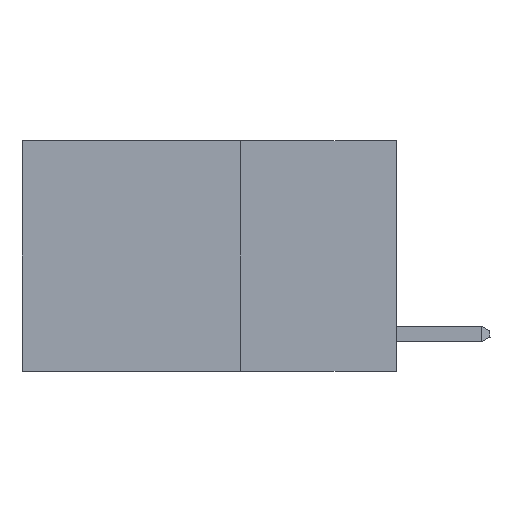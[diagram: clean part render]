
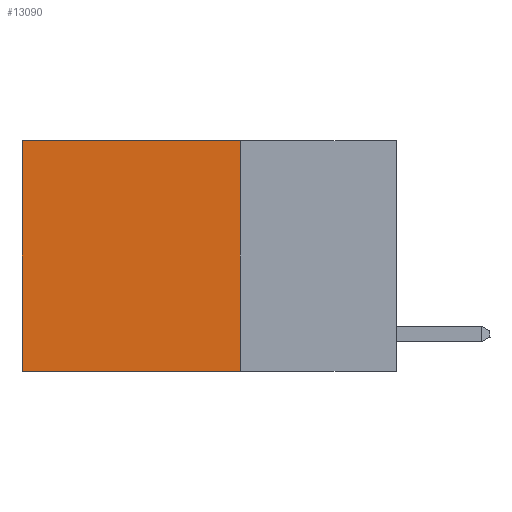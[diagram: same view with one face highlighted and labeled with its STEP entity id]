
A CAD part, left-side view. The second image highlights one B-rep face of the part: STEP entity #13090.
In plain terms, the highlighted planar face has unit normal (-1, 0, 0).
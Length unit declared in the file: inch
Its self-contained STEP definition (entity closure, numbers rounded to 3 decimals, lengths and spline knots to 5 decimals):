
#1786 = EDGE_CURVE ( 'NONE', #17122, #5156, #8942, .T. ) ;
#2832 = ORIENTED_EDGE ( 'NONE', *, *, #1786, .F. ) ;
#2873 = VECTOR ( 'NONE', #19897, 39.37008 ) ;
#3058 = LINE ( 'NONE', #7512, #3619 ) ;
#3619 = VECTOR ( 'NONE', #20273, 39.37008 ) ;
#3676 = CARTESIAN_POINT ( 'NONE',  ( 0.2625, 0.25, 0. ) ) ;
#3737 = VERTEX_POINT ( 'NONE', #13297 ) ;
#4144 = CARTESIAN_POINT ( 'NONE',  ( 0.2625, 0.25, 0. ) ) ;
#4507 = VECTOR ( 'NONE', #12484, 39.37008 ) ;
#5156 = VERTEX_POINT ( 'NONE', #11385 ) ;
#7353 = LINE ( 'NONE', #3676, #2873 ) ;
#7491 = DIRECTION ( 'NONE',  ( 0., 0., -1. ) ) ;
#7512 = CARTESIAN_POINT ( 'NONE',  ( 0.2625, 0.6, 0. ) ) ;
#7593 = VECTOR ( 'NONE', #7491, 39.37008 ) ;
#8550 = DIRECTION ( 'NONE',  ( 1., 0., 0. ) ) ;
#8942 = LINE ( 'NONE', #10857, #4507 ) ;
#10551 = CARTESIAN_POINT ( 'NONE',  ( 0.2625, 0.25, 0. ) ) ;
#10857 = CARTESIAN_POINT ( 'NONE',  ( 0.2625, 0.25, -0.37 ) ) ;
#11159 = ORIENTED_EDGE ( 'NONE', *, *, #13392, .T. ) ;
#11385 = CARTESIAN_POINT ( 'NONE',  ( 0.2625, 0.6, -0.37 ) ) ;
#11664 = ORIENTED_EDGE ( 'NONE', *, *, #11959, .F. ) ;
#11944 = LINE ( 'NONE', #4144, #7593 ) ;
#11959 = EDGE_CURVE ( 'NONE', #16475, #17122, #11944, .T. ) ;
#12484 = DIRECTION ( 'NONE',  ( 0., 1., 0. ) ) ;
#13090 = ADVANCED_FACE ( 'NONE', ( #13167 ), #18098, .F. ) ;
#13167 = FACE_OUTER_BOUND ( 'NONE', #14002, .T. ) ;
#13297 = CARTESIAN_POINT ( 'NONE',  ( 0.2625, 0.6, 0. ) ) ;
#13392 = EDGE_CURVE ( 'NONE', #3737, #5156, #3058, .T. ) ;
#14002 = EDGE_LOOP ( 'NONE', ( #11159, #2832, #11664, #20062 ) ) ;
#16475 = VERTEX_POINT ( 'NONE', #10551 ) ;
#17122 = VERTEX_POINT ( 'NONE', #19934 ) ;
#18098 = PLANE ( 'NONE',  #18361 ) ;
#18361 = AXIS2_PLACEMENT_3D ( 'NONE', #21175, #8550, #19676 ) ;
#18872 = EDGE_CURVE ( 'NONE', #16475, #3737, #7353, .T. ) ;
#19676 = DIRECTION ( 'NONE',  ( 0., 0., -1. ) ) ;
#19897 = DIRECTION ( 'NONE',  ( 0., 1., 0. ) ) ;
#19934 = CARTESIAN_POINT ( 'NONE',  ( 0.2625, 0.25, -0.37 ) ) ;
#20062 = ORIENTED_EDGE ( 'NONE', *, *, #18872, .T. ) ;
#20273 = DIRECTION ( 'NONE',  ( 0., 0., -1. ) ) ;
#21175 = CARTESIAN_POINT ( 'NONE',  ( 0.2625, 0.25, 0. ) ) ;
